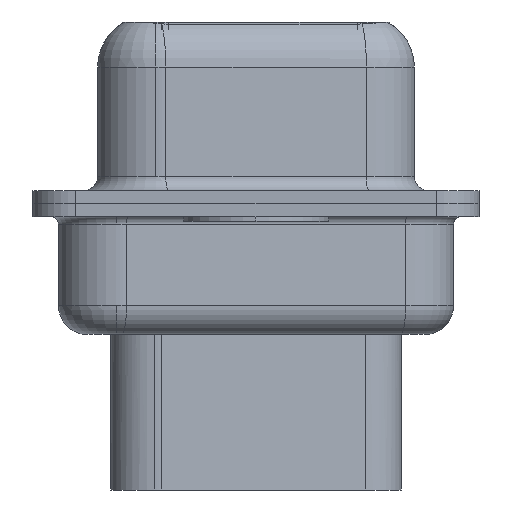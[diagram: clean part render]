
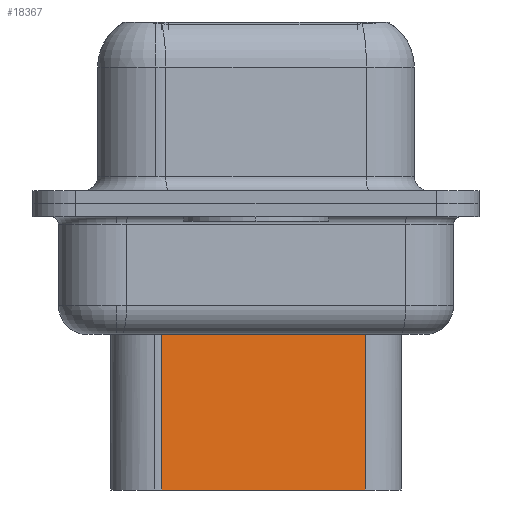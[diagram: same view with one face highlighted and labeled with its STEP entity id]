
A CAD part, left-side view. The second image highlights one B-rep face of the part: STEP entity #18367.
In plain terms, the highlighted planar face has unit normal (-0.985, -0.174, 0).
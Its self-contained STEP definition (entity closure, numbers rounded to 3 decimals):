
#430 = EDGE_CURVE ( 'NONE', #23506, #26412, #20137, .T. ) ;
#543 = CARTESIAN_POINT ( 'NONE',  ( 4.624, 3.24, -9.85 ) ) ;
#1032 = CARTESIAN_POINT ( 'NONE',  ( 4.624, 3.24, -9.85 ) ) ;
#2169 = VERTEX_POINT ( 'NONE', #35377 ) ;
#5548 = EDGE_CURVE ( 'NONE', #19374, #23506, #30487, .T. ) ;
#5851 = LINE ( 'NONE', #30162, #28861 ) ;
#6114 = LINE ( 'NONE', #33873, #34280 ) ;
#6666 = ORIENTED_EDGE ( 'NONE', *, *, #21678, .T. ) ;
#6932 = AXIS2_PLACEMENT_3D ( 'NONE', #27988, #34634, #15061 ) ;
#7383 = VECTOR ( 'NONE', #11589, 1000. ) ;
#11589 = DIRECTION ( 'NONE',  ( -0.174, 0.985, 0. ) ) ;
#12484 = PLANE ( 'NONE',  #6932 ) ;
#15061 = DIRECTION ( 'NONE',  ( 0.174, -0.985, 0. ) ) ;
#16524 = CARTESIAN_POINT ( 'NONE',  ( 5.858, -3.76, -3.1 ) ) ;
#16714 = DIRECTION ( 'NONE',  ( 0., 0., -1. ) ) ;
#16929 = DIRECTION ( 'NONE',  ( -0.174, 0.985, 0. ) ) ;
#16938 = FACE_OUTER_BOUND ( 'NONE', #31577, .T. ) ;
#18367 = ADVANCED_FACE ( 'NONE', ( #16938 ), #12484, .T. ) ;
#19374 = VERTEX_POINT ( 'NONE', #32596 ) ;
#20137 = LINE ( 'NONE', #543, #7383 ) ;
#20866 = EDGE_CURVE ( 'NONE', #2169, #26412, #6114, .T. ) ;
#21678 = EDGE_CURVE ( 'NONE', #19374, #2169, #5851, .T. ) ;
#23400 = VECTOR ( 'NONE', #16714, 1000. ) ;
#23506 = VERTEX_POINT ( 'NONE', #32221 ) ;
#24058 = ORIENTED_EDGE ( 'NONE', *, *, #430, .F. ) ;
#26412 = VERTEX_POINT ( 'NONE', #1032 ) ;
#27465 = ORIENTED_EDGE ( 'NONE', *, *, #5548, .F. ) ;
#27522 = DIRECTION ( 'NONE',  ( 0., 0., -1. ) ) ;
#27988 = CARTESIAN_POINT ( 'NONE',  ( 4.624, 3.24, -3.1 ) ) ;
#28861 = VECTOR ( 'NONE', #16929, 1000. ) ;
#29471 = ORIENTED_EDGE ( 'NONE', *, *, #20866, .T. ) ;
#30162 = CARTESIAN_POINT ( 'NONE',  ( 4.453, 4.209, -3.975 ) ) ;
#30487 = LINE ( 'NONE', #16524, #23400 ) ;
#31577 = EDGE_LOOP ( 'NONE', ( #27465, #6666, #29471, #24058 ) ) ;
#32221 = CARTESIAN_POINT ( 'NONE',  ( 5.858, -3.76, -9.85 ) ) ;
#32596 = CARTESIAN_POINT ( 'NONE',  ( 5.858, -3.76, -3.975 ) ) ;
#33873 = CARTESIAN_POINT ( 'NONE',  ( 4.624, 3.24, -3.1 ) ) ;
#34280 = VECTOR ( 'NONE', #27522, 1000. ) ;
#34634 = DIRECTION ( 'NONE',  ( -0.985, -0.174, 0. ) ) ;
#35377 = CARTESIAN_POINT ( 'NONE',  ( 4.624, 3.24, -3.975 ) ) ;
